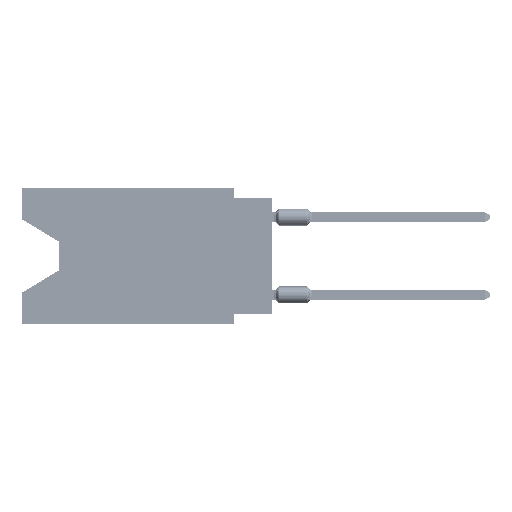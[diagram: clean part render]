
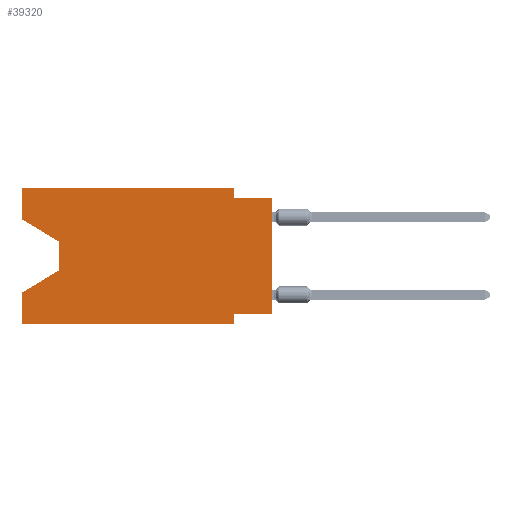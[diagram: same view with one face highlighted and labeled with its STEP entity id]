
A CAD part, left-side view. The second image highlights one B-rep face of the part: STEP entity #39320.
In plain terms, the highlighted planar face has unit normal (-1, 0, 0).
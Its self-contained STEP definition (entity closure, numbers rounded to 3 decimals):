
#402 = LINE ( 'NONE', #81361, #120070 ) ;
#2883 = CARTESIAN_POINT ( 'NONE',  ( 0., 0., 0. ) ) ;
#3246 = VECTOR ( 'NONE', #91014, 1000. ) ;
#4677 = CARTESIAN_POINT ( 'NONE',  ( 0., 16.383, 0. ) ) ;
#5795 = VECTOR ( 'NONE', #113591, 1000. ) ;
#5880 = CARTESIAN_POINT ( 'NONE',  ( 0., 2.54, -8.89 ) ) ;
#6298 = LINE ( 'NONE', #37088, #68733 ) ;
#11524 = ORIENTED_EDGE ( 'NONE', *, *, #72851, .T. ) ;
#14343 = ORIENTED_EDGE ( 'NONE', *, *, #69886, .F. ) ;
#15061 = VERTEX_POINT ( 'NONE', #19400 ) ;
#16221 = DIRECTION ( 'NONE',  ( 0., 0., -1. ) ) ;
#18281 = VERTEX_POINT ( 'NONE', #89460 ) ;
#18408 = LINE ( 'NONE', #22440, #99375 ) ;
#18666 = VERTEX_POINT ( 'NONE', #21654 ) ;
#18872 = VECTOR ( 'NONE', #34201, 1000. ) ;
#19400 = CARTESIAN_POINT ( 'NONE',  ( 0., 13.97, -5.385 ) ) ;
#21654 = CARTESIAN_POINT ( 'NONE',  ( 0., 16.383, -8.89 ) ) ;
#22440 = CARTESIAN_POINT ( 'NONE',  ( 0., 13.97, -5.385 ) ) ;
#23287 = LINE ( 'NONE', #60405, #18872 ) ;
#23650 = ORIENTED_EDGE ( 'NONE', *, *, #40086, .F. ) ;
#26542 = EDGE_CURVE ( 'NONE', #18666, #77683, #6298, .T. ) ;
#26565 = CARTESIAN_POINT ( 'NONE',  ( 0., 2.54, -8.89 ) ) ;
#30101 = ORIENTED_EDGE ( 'NONE', *, *, #120250, .F. ) ;
#30129 = LINE ( 'NONE', #31926, #58517 ) ;
#31926 = CARTESIAN_POINT ( 'NONE',  ( 0., 16.383, 0. ) ) ;
#33410 = EDGE_CURVE ( 'NONE', #34950, #49267, #86248, .T. ) ;
#33728 = VECTOR ( 'NONE', #81955, 1000. ) ;
#34201 = DIRECTION ( 'NONE',  ( 0., -1., 0. ) ) ;
#34417 = PLANE ( 'NONE',  #89859 ) ;
#34824 = VECTOR ( 'NONE', #46232, 1000. ) ;
#34950 = VERTEX_POINT ( 'NONE', #112873 ) ;
#35014 = EDGE_CURVE ( 'NONE', #112501, #75397, #30129, .T. ) ;
#35100 = ORIENTED_EDGE ( 'NONE', *, *, #35014, .F. ) ;
#37088 = CARTESIAN_POINT ( 'NONE',  ( 0., 16.383, 0. ) ) ;
#37093 = CARTESIAN_POINT ( 'NONE',  ( 0., 16.383, -2.038 ) ) ;
#37923 = VERTEX_POINT ( 'NONE', #112954 ) ;
#38092 = LINE ( 'NONE', #38686, #83206 ) ;
#38686 = CARTESIAN_POINT ( 'NONE',  ( 0., 0., -8.255 ) ) ;
#39320 = ADVANCED_FACE ( 'NONE', ( #79477 ), #34417, .F. ) ;
#39960 = DIRECTION ( 'NONE',  ( 0., -1., 0. ) ) ;
#40086 = EDGE_CURVE ( 'NONE', #92663, #115778, #79500, .T. ) ;
#41437 = EDGE_LOOP ( 'NONE', ( #11524, #114243, #74363, #109378, #108062, #23650, #30101, #66873, #108910, #14343, #72963, #35100 ) ) ;
#41460 = VECTOR ( 'NONE', #16221, 1000. ) ;
#46232 = DIRECTION ( 'NONE',  ( 0., -0.855, -0.519 ) ) ;
#46590 = VECTOR ( 'NONE', #39960, 1000. ) ;
#48380 = EDGE_CURVE ( 'NONE', #75397, #18281, #86233, .T. ) ;
#49267 = VERTEX_POINT ( 'NONE', #88789 ) ;
#49733 = CARTESIAN_POINT ( 'NONE',  ( 0., 2.54, -0.635 ) ) ;
#52399 = EDGE_CURVE ( 'NONE', #15061, #77683, #18408, .T. ) ;
#58517 = VECTOR ( 'NONE', #104935, 1000. ) ;
#59082 = VERTEX_POINT ( 'NONE', #49733 ) ;
#60405 = CARTESIAN_POINT ( 'NONE',  ( 0., 0., -0.635 ) ) ;
#61662 = DIRECTION ( 'NONE',  ( 0., 0., 1. ) ) ;
#62413 = CARTESIAN_POINT ( 'NONE',  ( 0., 16.383, 0. ) ) ;
#62434 = CARTESIAN_POINT ( 'NONE',  ( 0., 2.54, 0. ) ) ;
#63894 = LINE ( 'NONE', #37093, #34824 ) ;
#64523 = EDGE_CURVE ( 'NONE', #37923, #15061, #73423, .T. ) ;
#66873 = ORIENTED_EDGE ( 'NONE', *, *, #33410, .T. ) ;
#68089 = DIRECTION ( 'NONE',  ( 0., 0.855, -0.519 ) ) ;
#68733 = VECTOR ( 'NONE', #61662, 1000. ) ;
#69886 = EDGE_CURVE ( 'NONE', #18281, #59082, #99507, .T. ) ;
#72851 = EDGE_CURVE ( 'NONE', #112501, #37923, #63894, .T. ) ;
#72963 = ORIENTED_EDGE ( 'NONE', *, *, #48380, .F. ) ;
#73423 = LINE ( 'NONE', #110499, #33728 ) ;
#74016 = DIRECTION ( 'NONE',  ( 0., -1., 0. ) ) ;
#74363 = ORIENTED_EDGE ( 'NONE', *, *, #52399, .T. ) ;
#74690 = CARTESIAN_POINT ( 'NONE',  ( 0., 2.54, -8.255 ) ) ;
#75223 = DIRECTION ( 'NONE',  ( 0., 1., 0. ) ) ;
#75397 = VERTEX_POINT ( 'NONE', #109434 ) ;
#77683 = VERTEX_POINT ( 'NONE', #102885 ) ;
#78070 = CARTESIAN_POINT ( 'NONE',  ( 0., 16.383, -2.038 ) ) ;
#79477 = FACE_OUTER_BOUND ( 'NONE', #41437, .T. ) ;
#79500 = LINE ( 'NONE', #5880, #41460 ) ;
#81361 = CARTESIAN_POINT ( 'NONE',  ( 0., 16.383, -8.89 ) ) ;
#81955 = DIRECTION ( 'NONE',  ( 0., 0., -1. ) ) ;
#83206 = VECTOR ( 'NONE', #75223, 1000. ) ;
#86233 = LINE ( 'NONE', #4677, #46590 ) ;
#86248 = LINE ( 'NONE', #2883, #5795 ) ;
#88789 = CARTESIAN_POINT ( 'NONE',  ( 0., 0., -0.635 ) ) ;
#89460 = CARTESIAN_POINT ( 'NONE',  ( 0., 2.54, 0. ) ) ;
#89859 = AXIS2_PLACEMENT_3D ( 'NONE', #62413, #117738, #90398 ) ;
#90398 = DIRECTION ( 'NONE',  ( 0., 0., -1. ) ) ;
#91014 = DIRECTION ( 'NONE',  ( 0., 0., -1. ) ) ;
#92663 = VERTEX_POINT ( 'NONE', #74690 ) ;
#99375 = VECTOR ( 'NONE', #68089, 1000. ) ;
#99507 = LINE ( 'NONE', #62434, #3246 ) ;
#100013 = EDGE_CURVE ( 'NONE', #59082, #49267, #23287, .T. ) ;
#102885 = CARTESIAN_POINT ( 'NONE',  ( 0., 16.383, -6.852 ) ) ;
#104935 = DIRECTION ( 'NONE',  ( 0., 0., 1. ) ) ;
#108062 = ORIENTED_EDGE ( 'NONE', *, *, #120115, .T. ) ;
#108910 = ORIENTED_EDGE ( 'NONE', *, *, #100013, .F. ) ;
#109378 = ORIENTED_EDGE ( 'NONE', *, *, #26542, .F. ) ;
#109434 = CARTESIAN_POINT ( 'NONE',  ( 0., 16.383, 0. ) ) ;
#110499 = CARTESIAN_POINT ( 'NONE',  ( 0., 13.97, -3.505 ) ) ;
#112501 = VERTEX_POINT ( 'NONE', #78070 ) ;
#112873 = CARTESIAN_POINT ( 'NONE',  ( 0., 0., -8.255 ) ) ;
#112954 = CARTESIAN_POINT ( 'NONE',  ( 0., 13.97, -3.505 ) ) ;
#113591 = DIRECTION ( 'NONE',  ( 0., 0., 1. ) ) ;
#114243 = ORIENTED_EDGE ( 'NONE', *, *, #64523, .T. ) ;
#115778 = VERTEX_POINT ( 'NONE', #26565 ) ;
#117738 = DIRECTION ( 'NONE',  ( 1., 0., 0. ) ) ;
#120070 = VECTOR ( 'NONE', #74016, 1000. ) ;
#120115 = EDGE_CURVE ( 'NONE', #18666, #115778, #402, .T. ) ;
#120250 = EDGE_CURVE ( 'NONE', #34950, #92663, #38092, .T. ) ;
